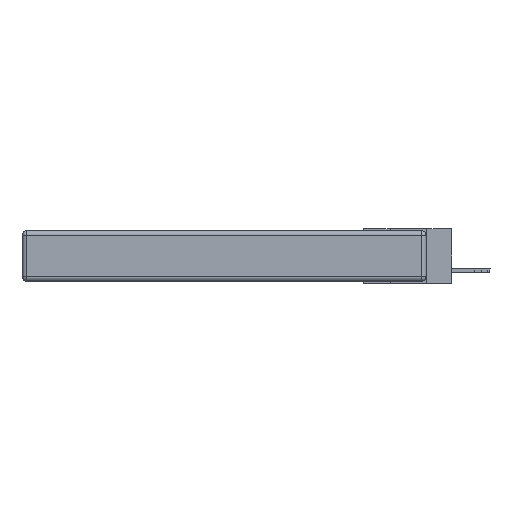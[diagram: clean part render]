
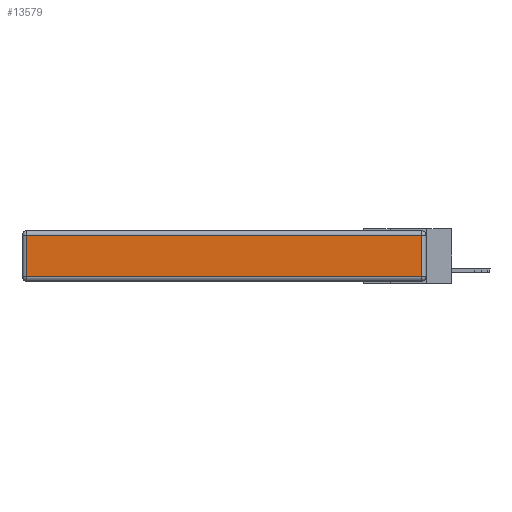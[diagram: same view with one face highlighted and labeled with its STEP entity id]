
A CAD part, left-side view. The second image highlights one B-rep face of the part: STEP entity #13579.
In plain terms, the highlighted planar face has unit normal (-1, 0, 0).
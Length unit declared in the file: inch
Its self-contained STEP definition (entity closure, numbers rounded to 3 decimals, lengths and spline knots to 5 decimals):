
#673 = CARTESIAN_POINT ( 'NONE',  ( 0., 0., -0.343 ) ) ;
#1439 = LINE ( 'NONE', #2466, #26916 ) ;
#2325 = CARTESIAN_POINT ( 'NONE',  ( 0., 0., -0.313 ) ) ;
#2357 = EDGE_LOOP ( 'NONE', ( #14814, #3436, #13424, #10047 ) ) ;
#2466 = CARTESIAN_POINT ( 'NONE',  ( 0., 2.72, -0.343 ) ) ;
#3344 = VECTOR ( 'NONE', #13039, 39.37008 ) ;
#3394 = CARTESIAN_POINT ( 'NONE',  ( 0., 0.03, -0.313 ) ) ;
#3436 = ORIENTED_EDGE ( 'NONE', *, *, #14148, .T. ) ;
#5537 = EDGE_CURVE ( 'NONE', #10176, #25275, #21757, .T. ) ;
#6314 = CARTESIAN_POINT ( 'NONE',  ( 0., 2.72, -0.03 ) ) ;
#6588 = FACE_OUTER_BOUND ( 'NONE', #2357, .T. ) ;
#7150 = DIRECTION ( 'NONE',  ( 0., 0., 1. ) ) ;
#8665 = DIRECTION ( 'NONE',  ( 0., 0., -1. ) ) ;
#9413 = DIRECTION ( 'NONE',  ( 0., 0., 1. ) ) ;
#10047 = ORIENTED_EDGE ( 'NONE', *, *, #15735, .T. ) ;
#10077 = LINE ( 'NONE', #22479, #24164 ) ;
#10176 = VERTEX_POINT ( 'NONE', #27748 ) ;
#11568 = DIRECTION ( 'NONE',  ( -1., 0., 0. ) ) ;
#11725 = VERTEX_POINT ( 'NONE', #3394 ) ;
#13039 = DIRECTION ( 'NONE',  ( 0., -1., 0. ) ) ;
#13424 = ORIENTED_EDGE ( 'NONE', *, *, #5537, .T. ) ;
#13579 = ADVANCED_FACE ( 'NONE', ( #6588 ), #16109, .T. ) ;
#13842 = VECTOR ( 'NONE', #21848, 39.37008 ) ;
#14148 = EDGE_CURVE ( 'NONE', #11725, #10176, #10077, .T. ) ;
#14814 = ORIENTED_EDGE ( 'NONE', *, *, #18380, .T. ) ;
#15091 = LINE ( 'NONE', #2325, #3344 ) ;
#15231 = CARTESIAN_POINT ( 'NONE',  ( 0., 2.75, -0.03 ) ) ;
#15735 = EDGE_CURVE ( 'NONE', #25275, #25877, #1439, .T. ) ;
#16109 = PLANE ( 'NONE',  #27266 ) ;
#18380 = EDGE_CURVE ( 'NONE', #25877, #11725, #15091, .T. ) ;
#21757 = LINE ( 'NONE', #15231, #13842 ) ;
#21848 = DIRECTION ( 'NONE',  ( 0., 1., 0. ) ) ;
#22479 = CARTESIAN_POINT ( 'NONE',  ( 0., 0.03, -0.343 ) ) ;
#24164 = VECTOR ( 'NONE', #9413, 39.37008 ) ;
#25275 = VERTEX_POINT ( 'NONE', #6314 ) ;
#25877 = VERTEX_POINT ( 'NONE', #28200 ) ;
#26916 = VECTOR ( 'NONE', #8665, 39.37008 ) ;
#27266 = AXIS2_PLACEMENT_3D ( 'NONE', #673, #11568, #7150 ) ;
#27748 = CARTESIAN_POINT ( 'NONE',  ( 0., 0.03, -0.03 ) ) ;
#28200 = CARTESIAN_POINT ( 'NONE',  ( 0., 2.72, -0.313 ) ) ;
